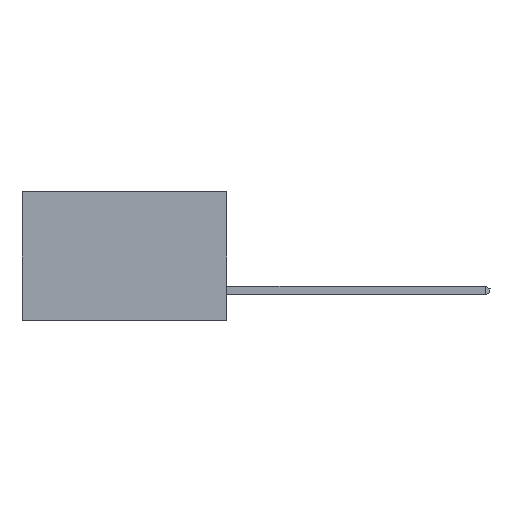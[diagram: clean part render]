
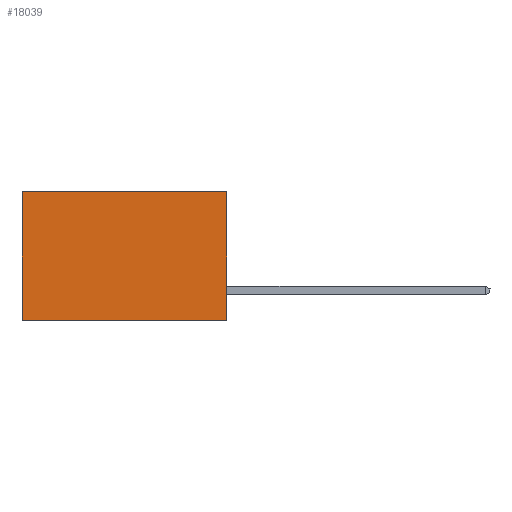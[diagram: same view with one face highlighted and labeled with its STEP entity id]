
A CAD part, left-side view. The second image highlights one B-rep face of the part: STEP entity #18039.
In plain terms, the highlighted planar face has unit normal (-1, 0, 0).
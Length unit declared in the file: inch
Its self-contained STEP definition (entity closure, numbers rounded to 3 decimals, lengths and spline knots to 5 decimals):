
#253 = CARTESIAN_POINT ( 'NONE',  ( 0.277, 0., -0.37 ) ) ;
#357 = CARTESIAN_POINT ( 'NONE',  ( 0.277, 0., -0.37 ) ) ;
#593 = EDGE_CURVE ( 'NONE', #12837, #1978, #6948, .T. ) ;
#875 = VECTOR ( 'NONE', #4530, 39.37008 ) ;
#1032 = VERTEX_POINT ( 'NONE', #26592 ) ;
#1676 = EDGE_CURVE ( 'NONE', #1978, #1032, #12874, .T. ) ;
#1978 = VERTEX_POINT ( 'NONE', #26769 ) ;
#3613 = VECTOR ( 'NONE', #24928, 39.37008 ) ;
#3938 = CARTESIAN_POINT ( 'NONE',  ( 0.277, 0., 0. ) ) ;
#4290 = PLANE ( 'NONE',  #13479 ) ;
#4530 = DIRECTION ( 'NONE',  ( 0., 0., -1. ) ) ;
#6438 = DIRECTION ( 'NONE',  ( 1., 0., 0. ) ) ;
#6809 = DIRECTION ( 'NONE',  ( 0., 1., 0. ) ) ;
#6948 = LINE ( 'NONE', #12940, #12594 ) ;
#7927 = CARTESIAN_POINT ( 'NONE',  ( 0.277, 0., -0.37 ) ) ;
#9485 = CARTESIAN_POINT ( 'NONE',  ( 0.277, 0.59, -0.37 ) ) ;
#11346 = EDGE_CURVE ( 'NONE', #12837, #24149, #20673, .T. ) ;
#12594 = VECTOR ( 'NONE', #12968, 39.37008 ) ;
#12651 = FACE_OUTER_BOUND ( 'NONE', #21150, .T. ) ;
#12837 = VERTEX_POINT ( 'NONE', #3938 ) ;
#12874 = LINE ( 'NONE', #9485, #875 ) ;
#12940 = CARTESIAN_POINT ( 'NONE',  ( 0.277, 0., 0. ) ) ;
#12968 = DIRECTION ( 'NONE',  ( 0., 1., 0. ) ) ;
#13479 = AXIS2_PLACEMENT_3D ( 'NONE', #19280, #6438, #21380 ) ;
#18039 = ADVANCED_FACE ( 'NONE', ( #12651 ), #4290, .F. ) ;
#19280 = CARTESIAN_POINT ( 'NONE',  ( 0.277, 0., -0.37 ) ) ;
#19787 = VECTOR ( 'NONE', #6809, 39.37008 ) ;
#20673 = LINE ( 'NONE', #7927, #3613 ) ;
#21150 = EDGE_LOOP ( 'NONE', ( #23142, #23302, #23637, #24396 ) ) ;
#21380 = DIRECTION ( 'NONE',  ( 0., 0., -1. ) ) ;
#21425 = EDGE_CURVE ( 'NONE', #24149, #1032, #25347, .T. ) ;
#23142 = ORIENTED_EDGE ( 'NONE', *, *, #1676, .T. ) ;
#23302 = ORIENTED_EDGE ( 'NONE', *, *, #21425, .F. ) ;
#23637 = ORIENTED_EDGE ( 'NONE', *, *, #11346, .F. ) ;
#24149 = VERTEX_POINT ( 'NONE', #253 ) ;
#24396 = ORIENTED_EDGE ( 'NONE', *, *, #593, .T. ) ;
#24928 = DIRECTION ( 'NONE',  ( 0., 0., -1. ) ) ;
#25347 = LINE ( 'NONE', #357, #19787 ) ;
#26592 = CARTESIAN_POINT ( 'NONE',  ( 0.277, 0.59, -0.37 ) ) ;
#26769 = CARTESIAN_POINT ( 'NONE',  ( 0.277, 0.59, 0. ) ) ;
